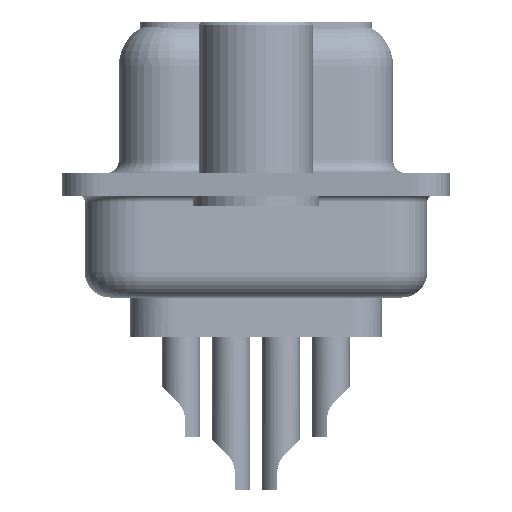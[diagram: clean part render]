
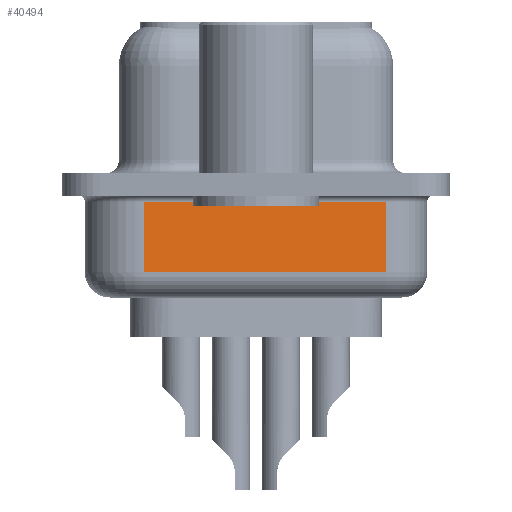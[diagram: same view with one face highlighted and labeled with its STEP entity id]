
A CAD part, left-side view. The second image highlights one B-rep face of the part: STEP entity #40494.
In plain terms, the highlighted planar face has unit normal (-0.985, -0.174, 0).
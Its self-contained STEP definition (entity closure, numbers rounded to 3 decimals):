
#108 = CARTESIAN_POINT ( 'NONE',  ( 4.728, -5.147, -0.7 ) ) ;
#669 = ORIENTED_EDGE ( 'NONE', *, *, #44242, .T. ) ;
#1406 = CARTESIAN_POINT ( 'NONE',  ( 3.035, 4.453, -0.7 ) ) ;
#3641 = VECTOR ( 'NONE', #48543, 1000. ) ;
#3794 = EDGE_CURVE ( 'NONE', #17113, #50552, #12503, .T. ) ;
#4509 = AXIS2_PLACEMENT_3D ( 'NONE', #5198, #21718, #46360 ) ;
#5198 = CARTESIAN_POINT ( 'NONE',  ( 3.035, 4.453, -4.5 ) ) ;
#6014 = LINE ( 'NONE', #18198, #27487 ) ;
#8545 = VERTEX_POINT ( 'NONE', #13626 ) ;
#12503 = LINE ( 'NONE', #16561, #3641 ) ;
#13626 = CARTESIAN_POINT ( 'NONE',  ( 3.035, 4.453, -0.7 ) ) ;
#16561 = CARTESIAN_POINT ( 'NONE',  ( 4.728, -5.147, -4.5 ) ) ;
#17113 = VERTEX_POINT ( 'NONE', #47291 ) ;
#18086 = VECTOR ( 'NONE', #25389, 1000. ) ;
#18198 = CARTESIAN_POINT ( 'NONE',  ( 3.035, 4.453, -4.5 ) ) ;
#18324 = ORIENTED_EDGE ( 'NONE', *, *, #43129, .T. ) ;
#18454 = PLANE ( 'NONE',  #4509 ) ;
#21718 = DIRECTION ( 'NONE',  ( 0.985, 0.174, 0. ) ) ;
#23068 = DIRECTION ( 'NONE',  ( -0.174, 0.985, 0. ) ) ;
#25389 = DIRECTION ( 'NONE',  ( 0.174, -0.985, 0. ) ) ;
#26582 = FACE_OUTER_BOUND ( 'NONE', #34768, .T. ) ;
#27487 = VECTOR ( 'NONE', #30394, 1000. ) ;
#29459 = LINE ( 'NONE', #49505, #18086 ) ;
#30394 = DIRECTION ( 'NONE',  ( 0., 0., 1. ) ) ;
#34398 = VECTOR ( 'NONE', #23068, 1000. ) ;
#34768 = EDGE_LOOP ( 'NONE', ( #40251, #669, #40723, #18324 ) ) ;
#38535 = LINE ( 'NONE', #1406, #34398 ) ;
#40251 = ORIENTED_EDGE ( 'NONE', *, *, #43059, .F. ) ;
#40494 = ADVANCED_FACE ( 'NONE', ( #26582 ), #18454, .F. ) ;
#40723 = ORIENTED_EDGE ( 'NONE', *, *, #3794, .T. ) ;
#43059 = EDGE_CURVE ( 'NONE', #51468, #8545, #6014, .T. ) ;
#43129 = EDGE_CURVE ( 'NONE', #50552, #8545, #38535, .T. ) ;
#44242 = EDGE_CURVE ( 'NONE', #51468, #17113, #29459, .T. ) ;
#46360 = DIRECTION ( 'NONE',  ( -0.174, 0.985, 0. ) ) ;
#47291 = CARTESIAN_POINT ( 'NONE',  ( 4.728, -5.147, -3.5 ) ) ;
#48388 = CARTESIAN_POINT ( 'NONE',  ( 3.035, 4.453, -3.5 ) ) ;
#48543 = DIRECTION ( 'NONE',  ( 0., 0., 1. ) ) ;
#49505 = CARTESIAN_POINT ( 'NONE',  ( 3.035, 4.453, -3.5 ) ) ;
#50552 = VERTEX_POINT ( 'NONE', #108 ) ;
#51468 = VERTEX_POINT ( 'NONE', #48388 ) ;
